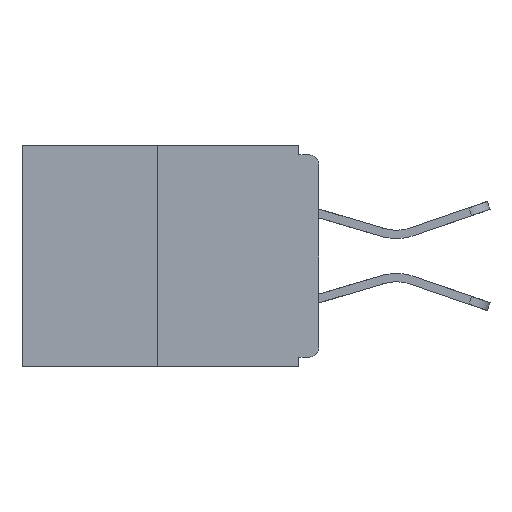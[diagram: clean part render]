
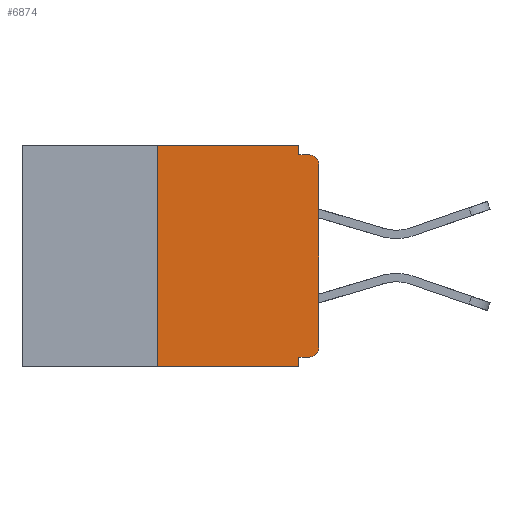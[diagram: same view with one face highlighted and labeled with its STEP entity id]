
A CAD part, left-side view. The second image highlights one B-rep face of the part: STEP entity #6874.
In plain terms, the highlighted planar face has unit normal (-1, 0, 0).
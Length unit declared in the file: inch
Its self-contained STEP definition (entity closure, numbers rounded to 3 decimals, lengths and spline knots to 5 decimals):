
#246 = DIRECTION ( 'NONE',  ( 0., 1., 0. ) ) ;
#411 = DIRECTION ( 'NONE',  ( 0., 0., 1. ) ) ;
#757 = AXIS2_PLACEMENT_3D ( 'NONE', #29296, #2052, #4537 ) ;
#1294 = LINE ( 'NONE', #20721, #22836 ) ;
#1417 = EDGE_CURVE ( 'NONE', #18882, #25062, #11969, .T. ) ;
#1976 = DIRECTION ( 'NONE',  ( 0., -1., 0. ) ) ;
#2052 = DIRECTION ( 'NONE',  ( -1., 0., 0. ) ) ;
#2601 = ORIENTED_EDGE ( 'NONE', *, *, #9149, .F. ) ;
#2675 = EDGE_LOOP ( 'NONE', ( #2601, #29953, #3078, #7075, #21906, #15654, #22951, #21884, #10159, #16862 ) ) ;
#3078 = ORIENTED_EDGE ( 'NONE', *, *, #6050, .T. ) ;
#3383 = VECTOR ( 'NONE', #28093, 39.37008 ) ;
#3413 = CARTESIAN_POINT ( 'NONE',  ( 0., 0.031, -0.015 ) ) ;
#3542 = VERTEX_POINT ( 'NONE', #30856 ) ;
#3631 = DIRECTION ( 'NONE',  ( 0., 0., -1. ) ) ;
#3758 = CIRCLE ( 'NONE', #757, 0.015 ) ;
#3923 = DIRECTION ( 'NONE',  ( 0., 0., -1. ) ) ;
#3941 = DIRECTION ( 'NONE',  ( 1., 0., 0. ) ) ;
#3973 = CARTESIAN_POINT ( 'NONE',  ( 0., 0.031, 0. ) ) ;
#4104 = VECTOR ( 'NONE', #246, 39.37008 ) ;
#4138 = DIRECTION ( 'NONE',  ( -1., 0., 0. ) ) ;
#4537 = DIRECTION ( 'NONE',  ( 0., 0., -1. ) ) ;
#5110 = VERTEX_POINT ( 'NONE', #28485 ) ;
#5845 = VECTOR ( 'NONE', #10981, 39.37008 ) ;
#5886 = FACE_OUTER_BOUND ( 'NONE', #2675, .T. ) ;
#6050 = EDGE_CURVE ( 'NONE', #18882, #8579, #1294, .T. ) ;
#6773 = DIRECTION ( 'NONE',  ( 0., 0., -1. ) ) ;
#6874 = ADVANCED_FACE ( 'NONE', ( #5886 ), #25749, .F. ) ;
#7075 = ORIENTED_EDGE ( 'NONE', *, *, #9921, .F. ) ;
#7189 = CARTESIAN_POINT ( 'NONE',  ( 0., 0.031, -0.328 ) ) ;
#8579 = VERTEX_POINT ( 'NONE', #21341 ) ;
#8611 = DIRECTION ( 'NONE',  ( 0., -1., 0. ) ) ;
#9086 = EDGE_CURVE ( 'NONE', #26147, #3542, #19197, .T. ) ;
#9149 = EDGE_CURVE ( 'NONE', #25062, #5110, #26081, .T. ) ;
#9488 = CARTESIAN_POINT ( 'NONE',  ( 0., 0.25, 0. ) ) ;
#9921 = EDGE_CURVE ( 'NONE', #23167, #8579, #26426, .T. ) ;
#10159 = ORIENTED_EDGE ( 'NONE', *, *, #27257, .F. ) ;
#10406 = EDGE_CURVE ( 'NONE', #26147, #23167, #16791, .T. ) ;
#10551 = CARTESIAN_POINT ( 'NONE',  ( 0., 0.25, 0. ) ) ;
#10981 = DIRECTION ( 'NONE',  ( 0., -1., 0. ) ) ;
#11728 = CARTESIAN_POINT ( 'NONE',  ( 0., 0.015, -0.015 ) ) ;
#11969 = LINE ( 'NONE', #10551, #25058 ) ;
#12761 = CARTESIAN_POINT ( 'NONE',  ( 0., 0., 0. ) ) ;
#14361 = LINE ( 'NONE', #12761, #26269 ) ;
#14627 = CARTESIAN_POINT ( 'NONE',  ( 0., 0.25, -0.343 ) ) ;
#15122 = CARTESIAN_POINT ( 'NONE',  ( 0., 0., -0.328 ) ) ;
#15368 = DIRECTION ( 'NONE',  ( 0., 0., 1. ) ) ;
#15654 = ORIENTED_EDGE ( 'NONE', *, *, #9086, .T. ) ;
#16294 = CARTESIAN_POINT ( 'NONE',  ( 0., 0.015, -0.313 ) ) ;
#16394 = VERTEX_POINT ( 'NONE', #3413 ) ;
#16791 = LINE ( 'NONE', #15122, #4104 ) ;
#16862 = ORIENTED_EDGE ( 'NONE', *, *, #22517, .F. ) ;
#17986 = CARTESIAN_POINT ( 'NONE',  ( 0., 0., -0.015 ) ) ;
#18178 = LINE ( 'NONE', #3973, #20494 ) ;
#18882 = VERTEX_POINT ( 'NONE', #14627 ) ;
#19197 = CIRCLE ( 'NONE', #25862, 0.015 ) ;
#19264 = AXIS2_PLACEMENT_3D ( 'NONE', #20728, #3941, #3631 ) ;
#20468 = LINE ( 'NONE', #17986, #5845 ) ;
#20494 = VECTOR ( 'NONE', #6773, 39.37008 ) ;
#20721 = CARTESIAN_POINT ( 'NONE',  ( 0., 0.46, -0.343 ) ) ;
#20728 = CARTESIAN_POINT ( 'NONE',  ( 0., 0.46, 0. ) ) ;
#21336 = CARTESIAN_POINT ( 'NONE',  ( 0., 0.46, 0. ) ) ;
#21341 = CARTESIAN_POINT ( 'NONE',  ( 0., 0.031, -0.343 ) ) ;
#21617 = EDGE_CURVE ( 'NONE', #3542, #23137, #14361, .T. ) ;
#21884 = ORIENTED_EDGE ( 'NONE', *, *, #30460, .T. ) ;
#21906 = ORIENTED_EDGE ( 'NONE', *, *, #10406, .F. ) ;
#22233 = VECTOR ( 'NONE', #1976, 39.37008 ) ;
#22517 = EDGE_CURVE ( 'NONE', #5110, #16394, #18178, .T. ) ;
#22836 = VECTOR ( 'NONE', #8611, 39.37008 ) ;
#22951 = ORIENTED_EDGE ( 'NONE', *, *, #21617, .T. ) ;
#23137 = VERTEX_POINT ( 'NONE', #28689 ) ;
#23167 = VERTEX_POINT ( 'NONE', #7189 ) ;
#23684 = VERTEX_POINT ( 'NONE', #11728 ) ;
#25058 = VECTOR ( 'NONE', #411, 39.37008 ) ;
#25062 = VERTEX_POINT ( 'NONE', #9488 ) ;
#25263 = CARTESIAN_POINT ( 'NONE',  ( 0., 0.031, -0.343 ) ) ;
#25749 = PLANE ( 'NONE',  #19264 ) ;
#25862 = AXIS2_PLACEMENT_3D ( 'NONE', #16294, #4138, #3923 ) ;
#26081 = LINE ( 'NONE', #21336, #22233 ) ;
#26147 = VERTEX_POINT ( 'NONE', #29099 ) ;
#26269 = VECTOR ( 'NONE', #15368, 39.37008 ) ;
#26426 = LINE ( 'NONE', #25263, #3383 ) ;
#27257 = EDGE_CURVE ( 'NONE', #16394, #23684, #20468, .T. ) ;
#28093 = DIRECTION ( 'NONE',  ( 0., 0., -1. ) ) ;
#28485 = CARTESIAN_POINT ( 'NONE',  ( 0., 0.031, 0. ) ) ;
#28689 = CARTESIAN_POINT ( 'NONE',  ( 0., 0., -0.03 ) ) ;
#29099 = CARTESIAN_POINT ( 'NONE',  ( 0., 0.015, -0.328 ) ) ;
#29296 = CARTESIAN_POINT ( 'NONE',  ( 0., 0.015, -0.03 ) ) ;
#29953 = ORIENTED_EDGE ( 'NONE', *, *, #1417, .F. ) ;
#30460 = EDGE_CURVE ( 'NONE', #23137, #23684, #3758, .T. ) ;
#30856 = CARTESIAN_POINT ( 'NONE',  ( 0., 0., -0.313 ) ) ;
